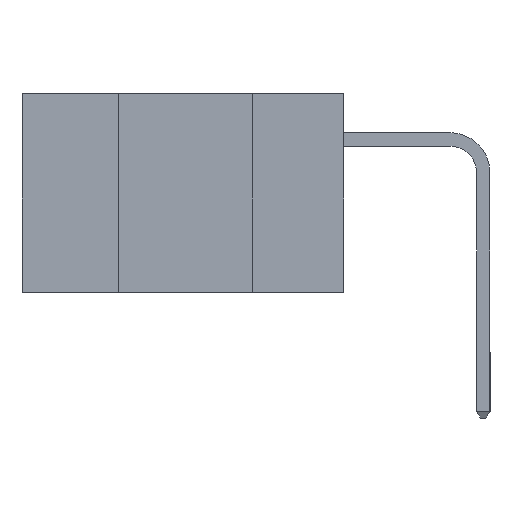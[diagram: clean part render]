
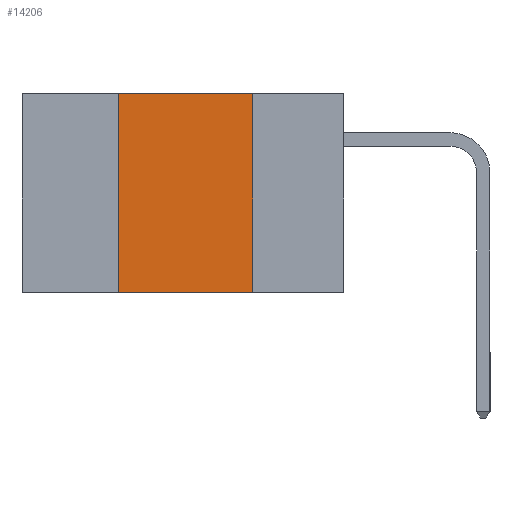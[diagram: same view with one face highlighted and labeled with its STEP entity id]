
A CAD part, left-side view. The second image highlights one B-rep face of the part: STEP entity #14206.
In plain terms, the highlighted planar face has unit normal (-1, 0, 0).
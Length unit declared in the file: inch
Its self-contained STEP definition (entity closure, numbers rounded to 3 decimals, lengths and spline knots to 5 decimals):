
#492 = CARTESIAN_POINT ( 'NONE',  ( 0., 0.17, 0. ) ) ;
#553 = EDGE_CURVE ( 'NONE', #2978, #4173, #3586, .T. ) ;
#788 = DIRECTION ( 'NONE',  ( 0., 0., -1. ) ) ;
#1489 = ORIENTED_EDGE ( 'NONE', *, *, #8000, .F. ) ;
#2715 = FACE_OUTER_BOUND ( 'NONE', #4050, .T. ) ;
#2821 = CARTESIAN_POINT ( 'NONE',  ( 0., 0.17, -0.37 ) ) ;
#2978 = VERTEX_POINT ( 'NONE', #492 ) ;
#3054 = VERTEX_POINT ( 'NONE', #3739 ) ;
#3344 = ORIENTED_EDGE ( 'NONE', *, *, #13873, .F. ) ;
#3517 = CARTESIAN_POINT ( 'NONE',  ( 0., 0.42, -0.37 ) ) ;
#3586 = LINE ( 'NONE', #8957, #6187 ) ;
#3739 = CARTESIAN_POINT ( 'NONE',  ( 0., 0.42, 0. ) ) ;
#4050 = EDGE_LOOP ( 'NONE', ( #9543, #3344, #1489, #8050 ) ) ;
#4125 = PLANE ( 'NONE',  #8248 ) ;
#4173 = VERTEX_POINT ( 'NONE', #2821 ) ;
#5129 = DIRECTION ( 'NONE',  ( 0., 0., 1. ) ) ;
#6187 = VECTOR ( 'NONE', #6627, 39.37008 ) ;
#6627 = DIRECTION ( 'NONE',  ( 0., 0., -1. ) ) ;
#6880 = VECTOR ( 'NONE', #5129, 39.37008 ) ;
#7055 = CARTESIAN_POINT ( 'NONE',  ( 0., 0.6, -0.37 ) ) ;
#8000 = EDGE_CURVE ( 'NONE', #12198, #3054, #9797, .T. ) ;
#8050 = ORIENTED_EDGE ( 'NONE', *, *, #14049, .T. ) ;
#8245 = LINE ( 'NONE', #11978, #13725 ) ;
#8248 = AXIS2_PLACEMENT_3D ( 'NONE', #11687, #10684, #788 ) ;
#8957 = CARTESIAN_POINT ( 'NONE',  ( 0., 0.17, 0. ) ) ;
#9543 = ORIENTED_EDGE ( 'NONE', *, *, #553, .F. ) ;
#9797 = LINE ( 'NONE', #13629, #6880 ) ;
#10684 = DIRECTION ( 'NONE',  ( 1., 0., 0. ) ) ;
#11488 = LINE ( 'NONE', #7055, #14232 ) ;
#11687 = CARTESIAN_POINT ( 'NONE',  ( 0., 0.6, 0. ) ) ;
#11978 = CARTESIAN_POINT ( 'NONE',  ( 0., 0.6, 0. ) ) ;
#12198 = VERTEX_POINT ( 'NONE', #3517 ) ;
#13527 = DIRECTION ( 'NONE',  ( 0., -1., 0. ) ) ;
#13629 = CARTESIAN_POINT ( 'NONE',  ( 0., 0.42, 0. ) ) ;
#13725 = VECTOR ( 'NONE', #14211, 39.37008 ) ;
#13873 = EDGE_CURVE ( 'NONE', #3054, #2978, #8245, .T. ) ;
#14049 = EDGE_CURVE ( 'NONE', #12198, #4173, #11488, .T. ) ;
#14206 = ADVANCED_FACE ( 'NONE', ( #2715 ), #4125, .F. ) ;
#14211 = DIRECTION ( 'NONE',  ( 0., -1., 0. ) ) ;
#14232 = VECTOR ( 'NONE', #13527, 39.37008 ) ;
